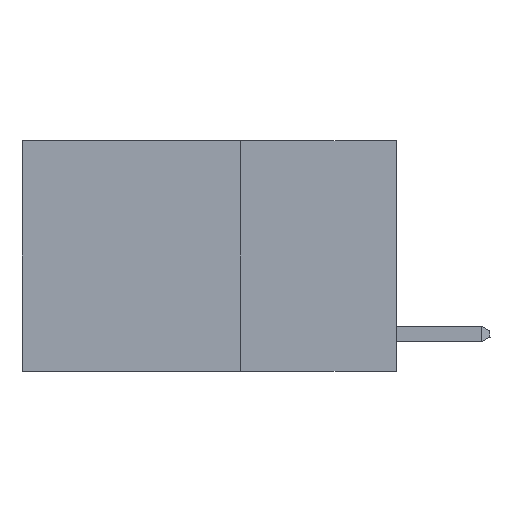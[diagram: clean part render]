
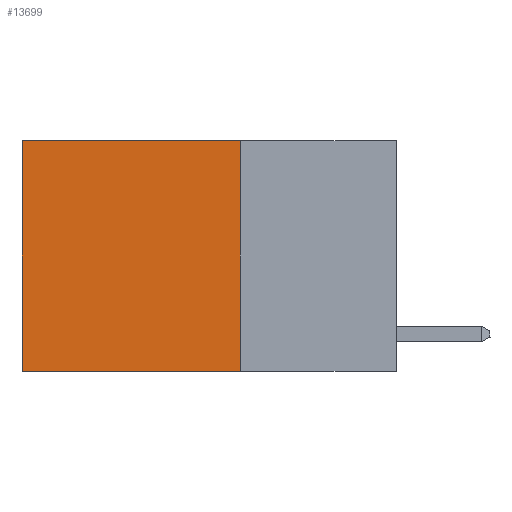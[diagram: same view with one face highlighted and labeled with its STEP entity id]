
A CAD part, left-side view. The second image highlights one B-rep face of the part: STEP entity #13699.
In plain terms, the highlighted planar face has unit normal (-1, 0, 0).
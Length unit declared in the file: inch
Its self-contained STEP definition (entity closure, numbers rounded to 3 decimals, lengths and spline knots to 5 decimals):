
#579 = FACE_OUTER_BOUND ( 'NONE', #23145, .T. ) ;
#1082 = DIRECTION ( 'NONE',  ( 0., 1., 0. ) ) ;
#1350 = ORIENTED_EDGE ( 'NONE', *, *, #3794, .T. ) ;
#1949 = LINE ( 'NONE', #9454, #11980 ) ;
#2041 = DIRECTION ( 'NONE',  ( 0., 1., 0. ) ) ;
#2437 = CARTESIAN_POINT ( 'NONE',  ( 0.2625, 0.25, 0. ) ) ;
#2820 = CARTESIAN_POINT ( 'NONE',  ( 0.2625, 0.25, -0.37 ) ) ;
#2974 = LINE ( 'NONE', #14437, #10524 ) ;
#3170 = EDGE_CURVE ( 'NONE', #14333, #16655, #1949, .T. ) ;
#3474 = VERTEX_POINT ( 'NONE', #2820 ) ;
#3738 = CARTESIAN_POINT ( 'NONE',  ( 0.2625, 0.6, -0.37 ) ) ;
#3794 = EDGE_CURVE ( 'NONE', #14101, #14333, #3929, .T. ) ;
#3929 = LINE ( 'NONE', #11897, #11622 ) ;
#6305 = DIRECTION ( 'NONE',  ( 0., 0., -1. ) ) ;
#8194 = DIRECTION ( 'NONE',  ( 1., 0., 0. ) ) ;
#8497 = ORIENTED_EDGE ( 'NONE', *, *, #14471, .F. ) ;
#9421 = DIRECTION ( 'NONE',  ( 0., 0., -1. ) ) ;
#9454 = CARTESIAN_POINT ( 'NONE',  ( 0.2625, 0.6, 0. ) ) ;
#10524 = VECTOR ( 'NONE', #1082, 39.37008 ) ;
#11276 = LINE ( 'NONE', #18909, #11893 ) ;
#11622 = VECTOR ( 'NONE', #2041, 39.37008 ) ;
#11893 = VECTOR ( 'NONE', #9421, 39.37008 ) ;
#11897 = CARTESIAN_POINT ( 'NONE',  ( 0.2625, 0.25, 0. ) ) ;
#11980 = VECTOR ( 'NONE', #19187, 39.37008 ) ;
#13333 = ORIENTED_EDGE ( 'NONE', *, *, #3170, .T. ) ;
#13699 = ADVANCED_FACE ( 'NONE', ( #579 ), #17825, .F. ) ;
#14101 = VERTEX_POINT ( 'NONE', #2437 ) ;
#14333 = VERTEX_POINT ( 'NONE', #23025 ) ;
#14437 = CARTESIAN_POINT ( 'NONE',  ( 0.2625, 0.25, -0.37 ) ) ;
#14471 = EDGE_CURVE ( 'NONE', #14101, #3474, #11276, .T. ) ;
#16655 = VERTEX_POINT ( 'NONE', #3738 ) ;
#17825 = PLANE ( 'NONE',  #22136 ) ;
#18177 = ORIENTED_EDGE ( 'NONE', *, *, #23718, .F. ) ;
#18909 = CARTESIAN_POINT ( 'NONE',  ( 0.2625, 0.25, 0. ) ) ;
#19187 = DIRECTION ( 'NONE',  ( 0., 0., -1. ) ) ;
#19807 = CARTESIAN_POINT ( 'NONE',  ( 0.2625, 0.25, 0. ) ) ;
#22136 = AXIS2_PLACEMENT_3D ( 'NONE', #19807, #8194, #6305 ) ;
#23025 = CARTESIAN_POINT ( 'NONE',  ( 0.2625, 0.6, 0. ) ) ;
#23145 = EDGE_LOOP ( 'NONE', ( #13333, #18177, #8497, #1350 ) ) ;
#23718 = EDGE_CURVE ( 'NONE', #3474, #16655, #2974, .T. ) ;
